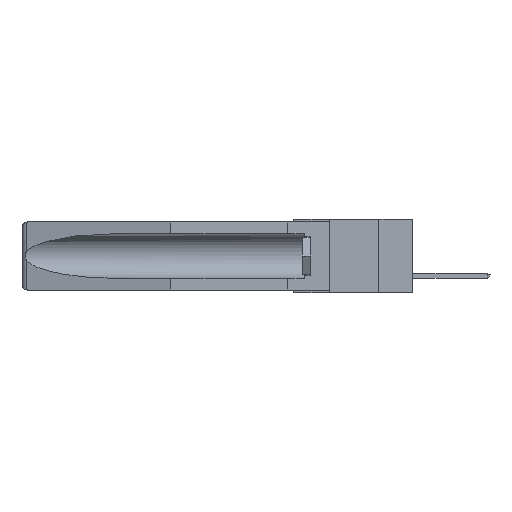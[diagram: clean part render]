
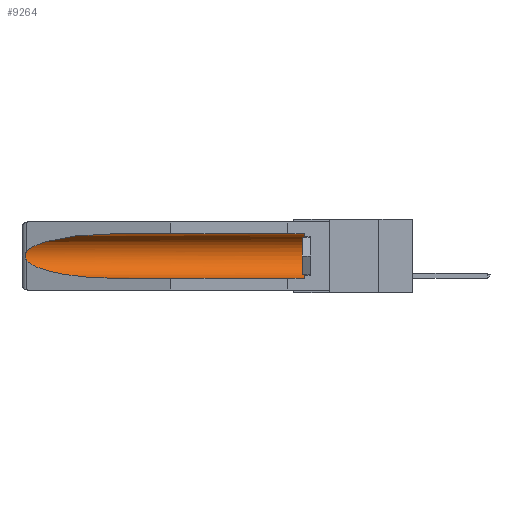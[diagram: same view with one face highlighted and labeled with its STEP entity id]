
A CAD part, left-side view. The second image highlights one B-rep face of the part: STEP entity #9264.
In plain terms, the highlighted cylindrical face has radius 2.857 mm (diameter 5.715 mm), a partial arc.
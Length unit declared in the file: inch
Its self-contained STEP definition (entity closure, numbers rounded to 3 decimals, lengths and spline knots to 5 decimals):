
#787 = CARTESIAN_POINT ( 'NONE',  ( 0.155, 0.126, -0.284 ) ) ;
#1539 = CARTESIAN_POINT ( 'NONE',  ( 0.2675, 1.53308, -0.17534 ) ) ;
#1616 = CARTESIAN_POINT ( 'NONE',  ( 0.155, -0.30754, -0.059 ) ) ;
#1817 = VERTEX_POINT ( 'NONE', #787 ) ;
#2003 = DIRECTION ( 'NONE',  ( 0., 0., 1. ) ) ;
#2146 = VERTEX_POINT ( 'NONE', #3803 ) ;
#2427 = VECTOR ( 'NONE', #15391, 39.37008 ) ;
#2918 = DIRECTION ( 'NONE',  ( 0., -1., 0. ) ) ;
#2935 = CARTESIAN_POINT ( 'NONE',  ( 0.26655, 1.53094, -0.18657 ) ) ;
#3070 = CARTESIAN_POINT ( 'NONE',  ( 0.26537, 1.52718, -0.14972 ) ) ;
#3081 = CARTESIAN_POINT ( 'NONE',  ( 0.26537, 1.52718, -0.14972 ) ) ;
#3437 = LINE ( 'NONE', #18530, #2427 ) ;
#3803 = CARTESIAN_POINT ( 'NONE',  ( 0.155, 1.07973, -0.284 ) ) ;
#4230 = EDGE_CURVE ( 'NONE', #4858, #17235, #11676, .T. ) ;
#4587 = CARTESIAN_POINT ( 'NONE',  ( 0.155, 1.07973, -0.059 ) ) ;
#4650 = CARTESIAN_POINT ( 'NONE',  ( 0.26597, 1.5296, -0.19026 ) ) ;
#4858 = VERTEX_POINT ( 'NONE', #11026 ) ;
#4866 = ORIENTED_EDGE ( 'NONE', *, *, #18274, .T. ) ;
#5620 = DIRECTION ( 'NONE',  ( 0., 1., 0. ) ) ;
#5697 = ORIENTED_EDGE ( 'NONE', *, *, #17222, .F. ) ;
#6165 = CARTESIAN_POINT ( 'NONE',  ( 0.2675, 1.53308, -0.16763 ) ) ;
#6541 = VERTEX_POINT ( 'NONE', #16981 ) ;
#6830 = CARTESIAN_POINT ( 'NONE',  ( 0.155, 0.126, -0.059 ) ) ;
#6848 = FACE_OUTER_BOUND ( 'NONE', #16666, .T. ) ;
#7484 = AXIS2_PLACEMENT_3D ( 'NONE', #12349, #2918, #17026 ) ;
#7757 = AXIS2_PLACEMENT_3D ( 'NONE', #19298, #9970, #2003 ) ;
#9264 = ADVANCED_FACE ( 'NONE', ( #6848 ), #16896, .F. ) ;
#9428 = CARTESIAN_POINT ( 'NONE',  ( 0.26537, 1.52718, -0.19328 ) ) ;
#9599 = ORIENTED_EDGE ( 'NONE', *, *, #9822, .T. ) ;
#9822 = EDGE_CURVE ( 'NONE', #11825, #6541, #12033, .T. ) ;
#9970 = DIRECTION ( 'NONE',  ( 0., 1., 0. ) ) ;
#10771 = CARTESIAN_POINT ( 'NONE',  ( 0.25451, 1.48313, -0.09465 ) ) ;
#10962 = CARTESIAN_POINT ( 'NONE',  ( 0.26654, 1.53092, -0.15636 ) ) ;
#11026 = CARTESIAN_POINT ( 'NONE',  ( 0.26537, 1.52718, -0.14972 ) ) ;
#11676 = B_SPLINE_CURVE_WITH_KNOTS ( 'NONE', 3,
 ( #3070, #17049, #10962, #12629, #6165, #1539, #18692, #2935, #4650, #9428 ),
 .UNSPECIFIED., .F., .F.,
 ( 4, 2, 2, 2, 4 ),
 ( 0., 0.00029, 0.00058, 0.00087, 0.00117 ),
 .UNSPECIFIED. ) ;
#11825 = VERTEX_POINT ( 'NONE', #6830 ) ;
#11991 = EDGE_CURVE ( 'NONE', #17235, #2146, #19415, .T. ) ;
#12033 = LINE ( 'NONE', #1616, #12517 ) ;
#12349 = CARTESIAN_POINT ( 'NONE',  ( 0.155, 0.126, -0.1715 ) ) ;
#12492 = CIRCLE ( 'NONE', #7484, 0.1125 ) ;
#12517 = VECTOR ( 'NONE', #5620, 39.37008 ) ;
#12629 = CARTESIAN_POINT ( 'NONE',  ( 0.2673, 1.5327, -0.16383 ) ) ;
#13674 = EDGE_CURVE ( 'NONE', #6541, #4858, #13886, .T. ) ;
#13886 =( BOUNDED_CURVE ( )  B_SPLINE_CURVE ( 3, ( #4587, #20070, #10771, #3081 ),
 .UNSPECIFIED., .F., .F. ) 
 B_SPLINE_CURVE_WITH_KNOTS ( ( 4, 4 ),
 ( 4.71239, 6.08839 ),
 .UNSPECIFIED. ) 
 CURVE ( )  GEOMETRIC_REPRESENTATION_ITEM ( )  RATIONAL_B_SPLINE_CURVE ( ( 1., 0.848, 0.848, 1. ) ) 
 REPRESENTATION_ITEM ( '' )  );
#15069 = CARTESIAN_POINT ( 'NONE',  ( 0.21114, 1.30732, -0.284 ) ) ;
#15391 = DIRECTION ( 'NONE',  ( 0., 1., 0. ) ) ;
#16620 = CARTESIAN_POINT ( 'NONE',  ( 0.155, 1.07973, -0.284 ) ) ;
#16666 = EDGE_LOOP ( 'NONE', ( #17895, #17065, #17845, #5697, #4866, #9599 ) ) ;
#16896 = CYLINDRICAL_SURFACE ( 'NONE', #7757, 0.1125 ) ;
#16981 = CARTESIAN_POINT ( 'NONE',  ( 0.155, 1.07973, -0.059 ) ) ;
#17026 = DIRECTION ( 'NONE',  ( 0., 0., 1. ) ) ;
#17049 = CARTESIAN_POINT ( 'NONE',  ( 0.26597, 1.52961, -0.15275 ) ) ;
#17065 = ORIENTED_EDGE ( 'NONE', *, *, #4230, .T. ) ;
#17222 = EDGE_CURVE ( 'NONE', #1817, #2146, #3437, .T. ) ;
#17235 = VERTEX_POINT ( 'NONE', #20026 ) ;
#17845 = ORIENTED_EDGE ( 'NONE', *, *, #11991, .T. ) ;
#17895 = ORIENTED_EDGE ( 'NONE', *, *, #13674, .T. ) ;
#18202 = CARTESIAN_POINT ( 'NONE',  ( 0.26537, 1.52718, -0.19328 ) ) ;
#18274 = EDGE_CURVE ( 'NONE', #1817, #11825, #12492, .T. ) ;
#18530 = CARTESIAN_POINT ( 'NONE',  ( 0.155, -0.30754, -0.284 ) ) ;
#18692 = CARTESIAN_POINT ( 'NONE',  ( 0.2673, 1.53269, -0.17917 ) ) ;
#19298 = CARTESIAN_POINT ( 'NONE',  ( 0.155, -0.30754, -0.1715 ) ) ;
#19415 =( BOUNDED_CURVE ( )  B_SPLINE_CURVE ( 3, ( #18202, #19703, #15069, #16620 ),
 .UNSPECIFIED., .F., .T. ) 
 B_SPLINE_CURVE_WITH_KNOTS ( ( 4, 4 ),
 ( 0.1948, 1.5708 ),
 .UNSPECIFIED. ) 
 CURVE ( )  GEOMETRIC_REPRESENTATION_ITEM ( )  RATIONAL_B_SPLINE_CURVE ( ( 1., 0.848, 0.848, 1. ) ) 
 REPRESENTATION_ITEM ( '' )  );
#19703 = CARTESIAN_POINT ( 'NONE',  ( 0.25451, 1.48313, -0.24835 ) ) ;
#20026 = CARTESIAN_POINT ( 'NONE',  ( 0.26537, 1.52718, -0.19328 ) ) ;
#20070 = CARTESIAN_POINT ( 'NONE',  ( 0.21114, 1.30732, -0.059 ) ) ;
